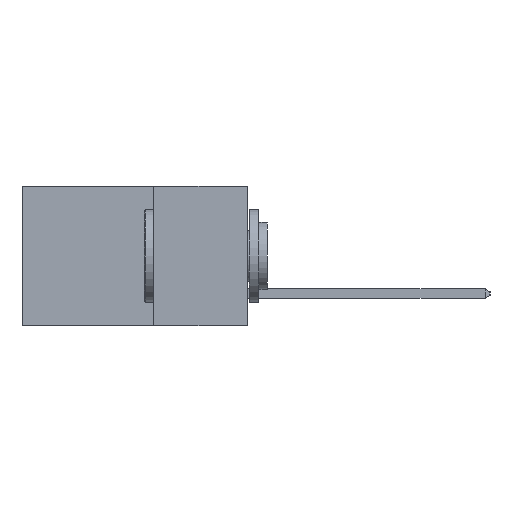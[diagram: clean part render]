
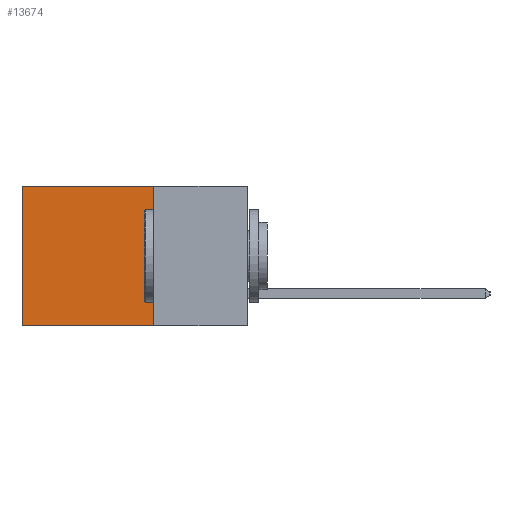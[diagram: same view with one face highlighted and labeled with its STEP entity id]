
A CAD part, left-side view. The second image highlights one B-rep face of the part: STEP entity #13674.
In plain terms, the highlighted planar face has unit normal (-1, 0, 0).
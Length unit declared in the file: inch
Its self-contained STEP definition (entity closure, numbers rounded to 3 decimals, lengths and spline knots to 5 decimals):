
#636 = CARTESIAN_POINT ( 'NONE',  ( 0.298, 0.25, 0. ) ) ;
#852 = ORIENTED_EDGE ( 'NONE', *, *, #5646, .F. ) ;
#2698 = CARTESIAN_POINT ( 'NONE',  ( 0.298, 0.6, -0.37 ) ) ;
#3215 = VERTEX_POINT ( 'NONE', #2698 ) ;
#4212 = VECTOR ( 'NONE', #7081, 39.37008 ) ;
#4980 = CARTESIAN_POINT ( 'NONE',  ( 0.298, 0.25, 0. ) ) ;
#5104 = VERTEX_POINT ( 'NONE', #26166 ) ;
#5646 = EDGE_CURVE ( 'NONE', #5104, #3215, #26032, .T. ) ;
#6187 = EDGE_CURVE ( 'NONE', #18330, #3215, #13630, .T. ) ;
#7081 = DIRECTION ( 'NONE',  ( 0., 1., 0. ) ) ;
#7407 = ORIENTED_EDGE ( 'NONE', *, *, #6187, .T. ) ;
#7424 = DIRECTION ( 'NONE',  ( 1., 0., 0. ) ) ;
#8688 = CARTESIAN_POINT ( 'NONE',  ( 0.298, 0.6, 0. ) ) ;
#9063 = DIRECTION ( 'NONE',  ( 0., 0., -1. ) ) ;
#9213 = FACE_OUTER_BOUND ( 'NONE', #11336, .T. ) ;
#10407 = VERTEX_POINT ( 'NONE', #26074 ) ;
#11027 = CARTESIAN_POINT ( 'NONE',  ( 0.298, 0.25, -0.37 ) ) ;
#11336 = EDGE_LOOP ( 'NONE', ( #7407, #852, #26057, #17723 ) ) ;
#11415 = EDGE_CURVE ( 'NONE', #10407, #18330, #20483, .T. ) ;
#11474 = PLANE ( 'NONE',  #15819 ) ;
#11757 = DIRECTION ( 'NONE',  ( 0., 1., 0. ) ) ;
#13630 = LINE ( 'NONE', #13790, #18351 ) ;
#13674 = ADVANCED_FACE ( 'NONE', ( #9213 ), #11474, .F. ) ;
#13790 = CARTESIAN_POINT ( 'NONE',  ( 0.298, 0.6, 0. ) ) ;
#14805 = EDGE_CURVE ( 'NONE', #10407, #5104, #22340, .T. ) ;
#15819 = AXIS2_PLACEMENT_3D ( 'NONE', #23446, #7424, #21601 ) ;
#17723 = ORIENTED_EDGE ( 'NONE', *, *, #11415, .T. ) ;
#18330 = VERTEX_POINT ( 'NONE', #8688 ) ;
#18351 = VECTOR ( 'NONE', #20627, 39.37008 ) ;
#20483 = LINE ( 'NONE', #4980, #4212 ) ;
#20627 = DIRECTION ( 'NONE',  ( 0., 0., -1. ) ) ;
#20863 = VECTOR ( 'NONE', #11757, 39.37008 ) ;
#21601 = DIRECTION ( 'NONE',  ( 0., 0., -1. ) ) ;
#21729 = VECTOR ( 'NONE', #9063, 39.37008 ) ;
#22340 = LINE ( 'NONE', #636, #21729 ) ;
#23446 = CARTESIAN_POINT ( 'NONE',  ( 0.298, 0.25, 0. ) ) ;
#26032 = LINE ( 'NONE', #11027, #20863 ) ;
#26057 = ORIENTED_EDGE ( 'NONE', *, *, #14805, .F. ) ;
#26074 = CARTESIAN_POINT ( 'NONE',  ( 0.298, 0.25, 0. ) ) ;
#26166 = CARTESIAN_POINT ( 'NONE',  ( 0.298, 0.25, -0.37 ) ) ;
